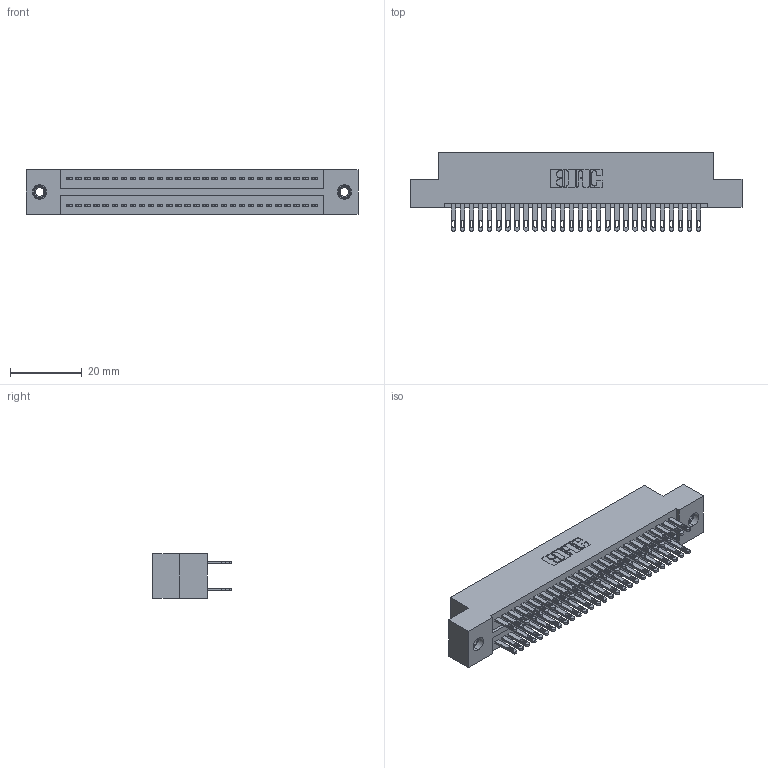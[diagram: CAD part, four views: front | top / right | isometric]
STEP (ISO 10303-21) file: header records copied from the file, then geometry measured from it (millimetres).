
FILE_DESCRIPTION (( 'STEP AP203' ), '1' );
FILE_NAME ('325-056-500-207.STEP', '2020-02-25T01:21:29', ( '' ), ( '' ), 'SwSTEP 2.0', 'SolidWorks 2016', '' );
FILE_SCHEMA (( 'CONFIG_CONTROL_DESIGN' ));
Length unit declared in the file: inch
Products named in the file (4): 345-250-001_345-250-005-103; 325 Part_TI; 325-056-500-207; 325-292-001_325-293-100
Assembly tree (59 placements, depth 2):
  325-056-500-207
    325 Part_TI
    325-292-001_325-293-100  x56
    345-250-001_345-250-005-103  x2
Bounding box: 92.84 x 21.84 x 12.45 mm (x, y, z)
Volume: 12016.8 mm3; surface area: 14824.6 mm2
Topology: 59 solids, 59 shells, 2862 faces, 8679 edges, 5778 vertices
Faces by surface type: plane 1782, cylinder 1064, cone 12, torus 4
Entity records: 20940 total; most frequent: CARTESIAN_POINT 3469, ORIENTED_EDGE 3398, DIRECTION 3021, EDGE_CURVE 1699, VECTOR 1547, LINE 1547, VERTEX_POINT 1128, AXIS2_PLACEMENT_3D 737
